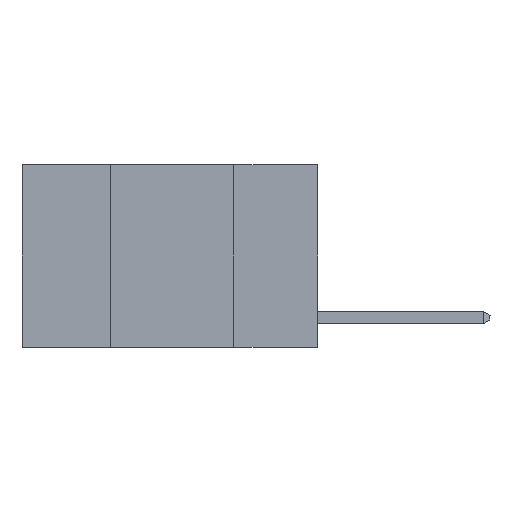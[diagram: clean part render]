
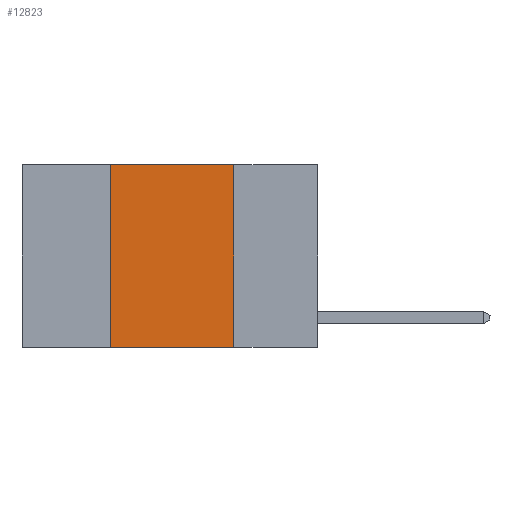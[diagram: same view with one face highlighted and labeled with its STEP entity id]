
A CAD part, left-side view. The second image highlights one B-rep face of the part: STEP entity #12823.
In plain terms, the highlighted planar face has unit normal (-1, 0, 0).
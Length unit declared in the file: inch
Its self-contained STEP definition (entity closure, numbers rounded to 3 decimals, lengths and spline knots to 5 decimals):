
#516 = CARTESIAN_POINT ( 'NONE',  ( 0., 0.42, 0. ) ) ;
#1367 = CARTESIAN_POINT ( 'NONE',  ( 0., 0.42, 0. ) ) ;
#1400 = VERTEX_POINT ( 'NONE', #11050 ) ;
#1993 = AXIS2_PLACEMENT_3D ( 'NONE', #9238, #7876, #15129 ) ;
#2313 = VECTOR ( 'NONE', #9823, 39.37008 ) ;
#2741 = LINE ( 'NONE', #1367, #2313 ) ;
#3197 = LINE ( 'NONE', #7810, #6819 ) ;
#3860 = ORIENTED_EDGE ( 'NONE', *, *, #5545, .F. ) ;
#4087 = VERTEX_POINT ( 'NONE', #516 ) ;
#4218 = ORIENTED_EDGE ( 'NONE', *, *, #8639, .F. ) ;
#4435 = CARTESIAN_POINT ( 'NONE',  ( 0., 0.17, 0. ) ) ;
#5545 = EDGE_CURVE ( 'NONE', #7718, #9660, #15195, .T. ) ;
#5613 = VECTOR ( 'NONE', #14931, 39.37008 ) ;
#6663 = CARTESIAN_POINT ( 'NONE',  ( 0., 0.6, -0.37 ) ) ;
#6819 = VECTOR ( 'NONE', #6877, 39.37008 ) ;
#6877 = DIRECTION ( 'NONE',  ( 0., -1., 0. ) ) ;
#7226 = EDGE_CURVE ( 'NONE', #1400, #4087, #2741, .T. ) ;
#7718 = VERTEX_POINT ( 'NONE', #12318 ) ;
#7810 = CARTESIAN_POINT ( 'NONE',  ( 0., 0.6, 0. ) ) ;
#7876 = DIRECTION ( 'NONE',  ( 1., 0., 0. ) ) ;
#8639 = EDGE_CURVE ( 'NONE', #4087, #7718, #3197, .T. ) ;
#9238 = CARTESIAN_POINT ( 'NONE',  ( 0., 0.6, 0. ) ) ;
#9319 = PLANE ( 'NONE',  #1993 ) ;
#9529 = CARTESIAN_POINT ( 'NONE',  ( 0., 0.17, -0.37 ) ) ;
#9556 = VECTOR ( 'NONE', #15117, 39.37008 ) ;
#9660 = VERTEX_POINT ( 'NONE', #9529 ) ;
#9823 = DIRECTION ( 'NONE',  ( 0., 0., 1. ) ) ;
#9957 = EDGE_CURVE ( 'NONE', #1400, #9660, #14772, .T. ) ;
#11050 = CARTESIAN_POINT ( 'NONE',  ( 0., 0.42, -0.37 ) ) ;
#12318 = CARTESIAN_POINT ( 'NONE',  ( 0., 0.17, 0. ) ) ;
#12546 = EDGE_LOOP ( 'NONE', ( #3860, #4218, #14954, #15376 ) ) ;
#12823 = ADVANCED_FACE ( 'NONE', ( #13954 ), #9319, .F. ) ;
#13954 = FACE_OUTER_BOUND ( 'NONE', #12546, .T. ) ;
#14772 = LINE ( 'NONE', #6663, #5613 ) ;
#14931 = DIRECTION ( 'NONE',  ( 0., -1., 0. ) ) ;
#14954 = ORIENTED_EDGE ( 'NONE', *, *, #7226, .F. ) ;
#15117 = DIRECTION ( 'NONE',  ( 0., 0., -1. ) ) ;
#15129 = DIRECTION ( 'NONE',  ( 0., 0., -1. ) ) ;
#15195 = LINE ( 'NONE', #4435, #9556 ) ;
#15376 = ORIENTED_EDGE ( 'NONE', *, *, #9957, .T. ) ;
